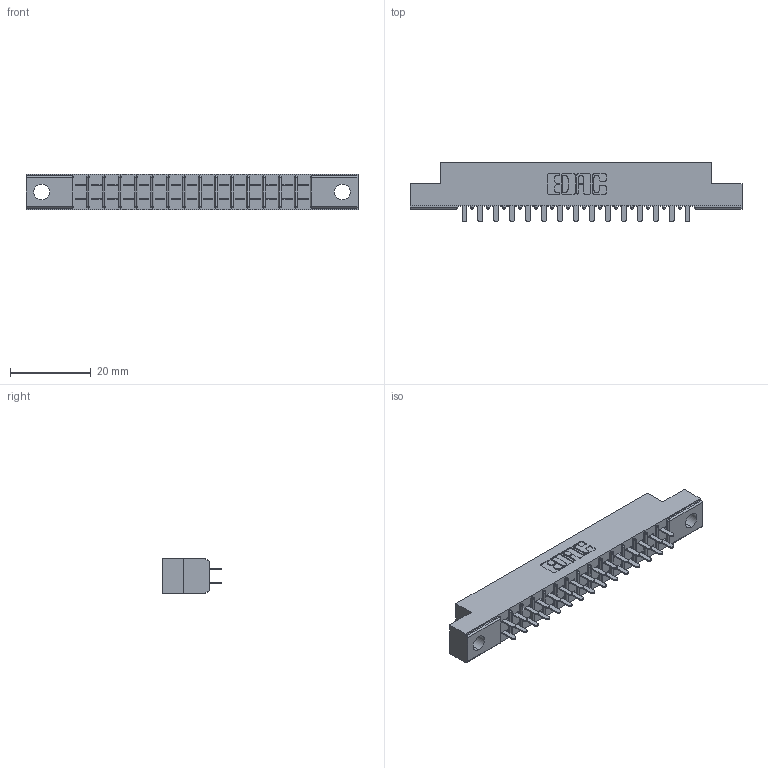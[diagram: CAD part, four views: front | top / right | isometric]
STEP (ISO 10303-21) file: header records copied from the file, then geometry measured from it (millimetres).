
FILE_DESCRIPTION (( 'STEP AP203' ), '1' );
FILE_NAME ('315-030-521-204.STEP', '2019-09-10T15:24:04', ( '' ), ( '' ), 'SwSTEP 2.0', 'SolidWorks 2016', '' );
FILE_SCHEMA (( 'CONFIG_CONTROL_DESIGN' ));
Length unit declared in the file: inch
Products named in the file (3): 305 Part_.156 Dia; 305-290-001_521; 315-030-521-204
Assembly tree (31 placements, depth 2):
  315-030-521-204
    305 Part_.156 Dia
    305-290-001_521  x30
Bounding box: 82.45 x 14.86 x 8.71 mm (x, y, z)
Volume: 5051.8 mm3; surface area: 8891.8 mm2
Topology: 31 solids, 31 shells, 1510 faces, 4297 edges, 2782 vertices
Faces by surface type: plane 892, cylinder 558, sphere 60
Entity records: 19826 total; most frequent: CARTESIAN_POINT 3285, ORIENTED_EDGE 3254, DIRECTION 3191, EDGE_CURVE 1627, VECTOR 1295, LINE 1295, VERTEX_POINT 1042, AXIS2_PLACEMENT_3D 948
